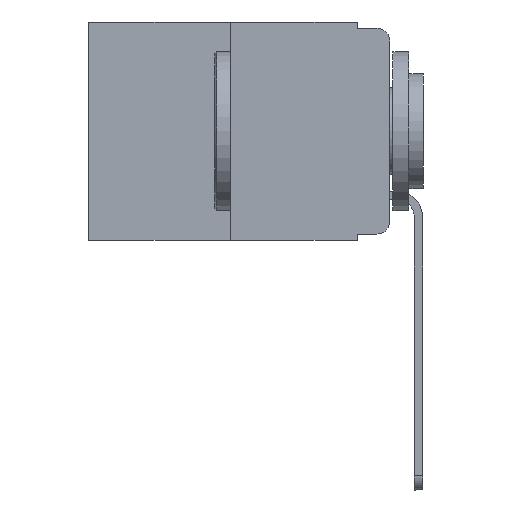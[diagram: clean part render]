
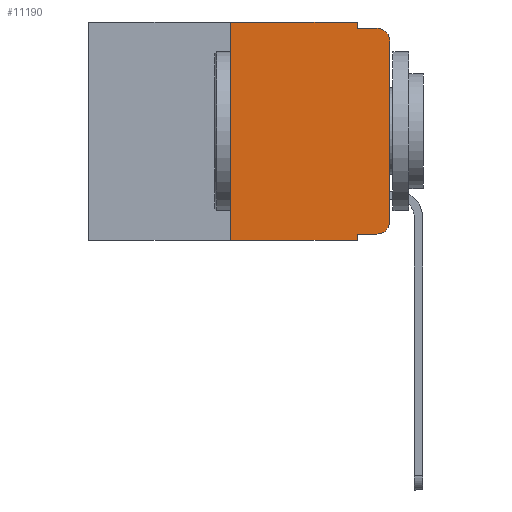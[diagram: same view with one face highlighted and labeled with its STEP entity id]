
A CAD part, left-side view. The second image highlights one B-rep face of the part: STEP entity #11190.
In plain terms, the highlighted planar face has unit normal (-1, 0, 0).
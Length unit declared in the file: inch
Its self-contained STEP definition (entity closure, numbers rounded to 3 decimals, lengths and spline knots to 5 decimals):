
#275 = ORIENTED_EDGE ( 'NONE', *, *, #10304, .F. ) ;
#314 = CIRCLE ( 'NONE', #13821, 0.02 ) ;
#1157 = CARTESIAN_POINT ( 'NONE',  ( 0., 0., -0.313 ) ) ;
#1267 = CARTESIAN_POINT ( 'NONE',  ( 0., 0.051, -0.01 ) ) ;
#1413 = DIRECTION ( 'NONE',  ( 1., 0., 0. ) ) ;
#1559 = LINE ( 'NONE', #4917, #7634 ) ;
#1655 = CARTESIAN_POINT ( 'NONE',  ( 0., 0.02, -0.313 ) ) ;
#1804 = DIRECTION ( 'NONE',  ( 0., 0., -1. ) ) ;
#1935 = CARTESIAN_POINT ( 'NONE',  ( 0., 0.02, -0.333 ) ) ;
#2056 = PLANE ( 'NONE',  #4094 ) ;
#2321 = CARTESIAN_POINT ( 'NONE',  ( 0., 0.051, 0. ) ) ;
#2494 = DIRECTION ( 'NONE',  ( 0., -1., 0. ) ) ;
#2526 = CIRCLE ( 'NONE', #11118, 0.02 ) ;
#3017 = LINE ( 'NONE', #8849, #14057 ) ;
#3177 = DIRECTION ( 'NONE',  ( 0., -1., 0. ) ) ;
#3235 = VERTEX_POINT ( 'NONE', #9560 ) ;
#3260 = CARTESIAN_POINT ( 'NONE',  ( 0., 0.473, 0. ) ) ;
#3335 = ORIENTED_EDGE ( 'NONE', *, *, #12640, .F. ) ;
#3581 = VECTOR ( 'NONE', #11673, 39.37008 ) ;
#3825 = EDGE_CURVE ( 'NONE', #3235, #10281, #5400, .T. ) ;
#4094 = AXIS2_PLACEMENT_3D ( 'NONE', #14583, #1413, #8464 ) ;
#4105 = VECTOR ( 'NONE', #5535, 39.37008 ) ;
#4191 = VECTOR ( 'NONE', #6402, 39.37008 ) ;
#4395 = CARTESIAN_POINT ( 'NONE',  ( 0., 0.02, -0.03 ) ) ;
#4643 = VERTEX_POINT ( 'NONE', #11272 ) ;
#4831 = EDGE_LOOP ( 'NONE', ( #12334, #10276, #10466, #3335, #11162, #275, #7517, #8587, #12294, #5734 ) ) ;
#4917 = CARTESIAN_POINT ( 'NONE',  ( 0., 0., 0. ) ) ;
#5400 = LINE ( 'NONE', #11093, #4191 ) ;
#5456 = VECTOR ( 'NONE', #12775, 39.37008 ) ;
#5498 = LINE ( 'NONE', #3260, #14536 ) ;
#5535 = DIRECTION ( 'NONE',  ( 0., 0., 1. ) ) ;
#5734 = ORIENTED_EDGE ( 'NONE', *, *, #12441, .T. ) ;
#6402 = DIRECTION ( 'NONE',  ( 0., -1., 0. ) ) ;
#6612 = CARTESIAN_POINT ( 'NONE',  ( 0., 0.25, 0. ) ) ;
#7295 = DIRECTION ( 'NONE',  ( 0., 0., 1. ) ) ;
#7517 = ORIENTED_EDGE ( 'NONE', *, *, #7525, .T. ) ;
#7525 = EDGE_CURVE ( 'NONE', #9652, #14544, #13976, .T. ) ;
#7634 = VECTOR ( 'NONE', #7295, 39.37008 ) ;
#7761 = VERTEX_POINT ( 'NONE', #8964 ) ;
#7871 = FACE_OUTER_BOUND ( 'NONE', #4831, .T. ) ;
#7980 = LINE ( 'NONE', #6612, #4105 ) ;
#8268 = EDGE_CURVE ( 'NONE', #14315, #8861, #9246, .T. ) ;
#8464 = DIRECTION ( 'NONE',  ( 0., 0., -1. ) ) ;
#8587 = ORIENTED_EDGE ( 'NONE', *, *, #12603, .F. ) ;
#8849 = CARTESIAN_POINT ( 'NONE',  ( 0., 0.051, 0. ) ) ;
#8861 = VERTEX_POINT ( 'NONE', #14537 ) ;
#8964 = CARTESIAN_POINT ( 'NONE',  ( 0., 0., -0.03 ) ) ;
#9011 = VECTOR ( 'NONE', #2494, 39.37008 ) ;
#9246 = LINE ( 'NONE', #1267, #9011 ) ;
#9299 = LINE ( 'NONE', #2321, #5456 ) ;
#9347 = CARTESIAN_POINT ( 'NONE',  ( 0., 0.473, -0.343 ) ) ;
#9560 = CARTESIAN_POINT ( 'NONE',  ( 0., 0.051, -0.333 ) ) ;
#9652 = VERTEX_POINT ( 'NONE', #11175 ) ;
#10276 = ORIENTED_EDGE ( 'NONE', *, *, #12531, .T. ) ;
#10281 = VERTEX_POINT ( 'NONE', #1935 ) ;
#10304 = EDGE_CURVE ( 'NONE', #9652, #12989, #7980, .T. ) ;
#10466 = ORIENTED_EDGE ( 'NONE', *, *, #8268, .F. ) ;
#11093 = CARTESIAN_POINT ( 'NONE',  ( 0., 0.051, -0.333 ) ) ;
#11118 = AXIS2_PLACEMENT_3D ( 'NONE', #4395, #13709, #14932 ) ;
#11162 = ORIENTED_EDGE ( 'NONE', *, *, #12144, .F. ) ;
#11175 = CARTESIAN_POINT ( 'NONE',  ( 0., 0.25, -0.343 ) ) ;
#11190 = ADVANCED_FACE ( 'NONE', ( #7871 ), #2056, .F. ) ;
#11272 = CARTESIAN_POINT ( 'NONE',  ( 0., 0.051, 0. ) ) ;
#11673 = DIRECTION ( 'NONE',  ( 0., -1., 0. ) ) ;
#11683 = CARTESIAN_POINT ( 'NONE',  ( 0., 0.051, -0.01 ) ) ;
#12144 = EDGE_CURVE ( 'NONE', #12989, #4643, #5498, .T. ) ;
#12294 = ORIENTED_EDGE ( 'NONE', *, *, #3825, .T. ) ;
#12326 = DIRECTION ( 'NONE',  ( -1., 0., 0. ) ) ;
#12334 = ORIENTED_EDGE ( 'NONE', *, *, #12884, .T. ) ;
#12441 = EDGE_CURVE ( 'NONE', #10281, #14325, #314, .T. ) ;
#12531 = EDGE_CURVE ( 'NONE', #7761, #8861, #2526, .T. ) ;
#12603 = EDGE_CURVE ( 'NONE', #3235, #14544, #3017, .T. ) ;
#12640 = EDGE_CURVE ( 'NONE', #4643, #14315, #9299, .T. ) ;
#12775 = DIRECTION ( 'NONE',  ( 0., 0., -1. ) ) ;
#12884 = EDGE_CURVE ( 'NONE', #14325, #7761, #1559, .T. ) ;
#12989 = VERTEX_POINT ( 'NONE', #13610 ) ;
#13557 = DIRECTION ( 'NONE',  ( 0., 0., -1. ) ) ;
#13610 = CARTESIAN_POINT ( 'NONE',  ( 0., 0.25, 0. ) ) ;
#13709 = DIRECTION ( 'NONE',  ( -1., 0., 0. ) ) ;
#13821 = AXIS2_PLACEMENT_3D ( 'NONE', #1655, #12326, #1804 ) ;
#13976 = LINE ( 'NONE', #9347, #3581 ) ;
#14057 = VECTOR ( 'NONE', #13557, 39.37008 ) ;
#14315 = VERTEX_POINT ( 'NONE', #11683 ) ;
#14325 = VERTEX_POINT ( 'NONE', #1157 ) ;
#14536 = VECTOR ( 'NONE', #3177, 39.37008 ) ;
#14537 = CARTESIAN_POINT ( 'NONE',  ( 0., 0.02, -0.01 ) ) ;
#14544 = VERTEX_POINT ( 'NONE', #14897 ) ;
#14583 = CARTESIAN_POINT ( 'NONE',  ( 0., 0.473, 0. ) ) ;
#14897 = CARTESIAN_POINT ( 'NONE',  ( 0., 0.051, -0.343 ) ) ;
#14932 = DIRECTION ( 'NONE',  ( 0., 0., -1. ) ) ;
